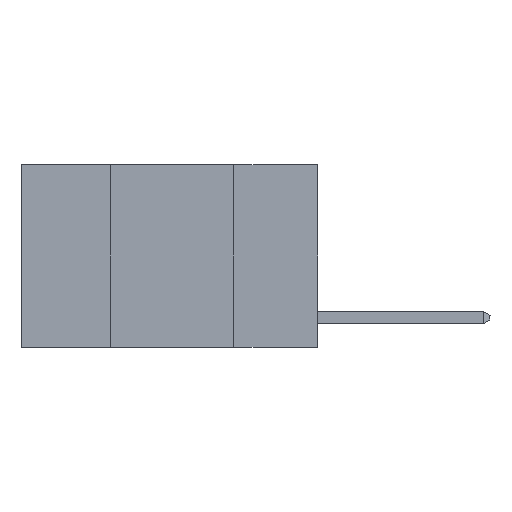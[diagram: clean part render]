
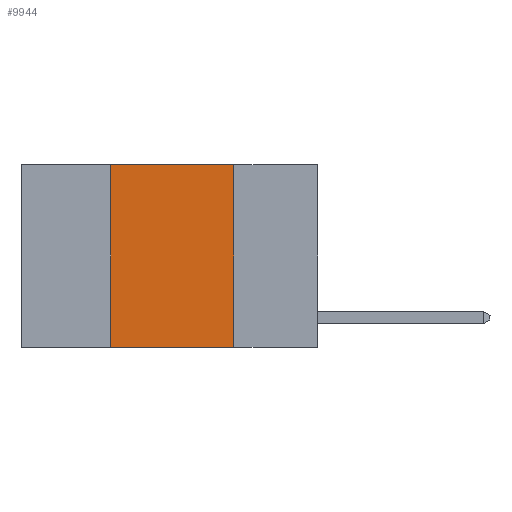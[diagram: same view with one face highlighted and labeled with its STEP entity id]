
A CAD part, left-side view. The second image highlights one B-rep face of the part: STEP entity #9944.
In plain terms, the highlighted planar face has unit normal (-1, 0, 0).
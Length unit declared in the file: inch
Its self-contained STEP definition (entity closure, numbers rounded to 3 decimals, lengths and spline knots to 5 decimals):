
#78 = EDGE_CURVE ( 'NONE', #9861, #7901, #6648, .T. ) ;
#279 = ORIENTED_EDGE ( 'NONE', *, *, #1181, .T. ) ;
#716 = CARTESIAN_POINT ( 'NONE',  ( 0., 0.6, 0. ) ) ;
#1181 = EDGE_CURVE ( 'NONE', #4732, #7901, #4963, .T. ) ;
#1214 = PLANE ( 'NONE',  #4737 ) ;
#1328 = EDGE_LOOP ( 'NONE', ( #4521, #8179, #10291, #279 ) ) ;
#1465 = CARTESIAN_POINT ( 'NONE',  ( 0., 0.42, -0.37 ) ) ;
#1724 = DIRECTION ( 'NONE',  ( 0., -1., 0. ) ) ;
#1966 = DIRECTION ( 'NONE',  ( 0., 0., -1. ) ) ;
#2116 = DIRECTION ( 'NONE',  ( 1., 0., 0. ) ) ;
#2265 = EDGE_CURVE ( 'NONE', #4308, #9861, #6457, .T. ) ;
#2433 = VECTOR ( 'NONE', #10717, 39.37008 ) ;
#2721 = VECTOR ( 'NONE', #1724, 39.37008 ) ;
#3752 = VECTOR ( 'NONE', #5620, 39.37008 ) ;
#3989 = FACE_OUTER_BOUND ( 'NONE', #1328, .T. ) ;
#4106 = CARTESIAN_POINT ( 'NONE',  ( 0., 0.6, 0. ) ) ;
#4308 = VERTEX_POINT ( 'NONE', #8028 ) ;
#4517 = VECTOR ( 'NONE', #1966, 39.37008 ) ;
#4521 = ORIENTED_EDGE ( 'NONE', *, *, #78, .F. ) ;
#4732 = VERTEX_POINT ( 'NONE', #1465 ) ;
#4737 = AXIS2_PLACEMENT_3D ( 'NONE', #4106, #2116, #8637 ) ;
#4963 = LINE ( 'NONE', #9739, #2433 ) ;
#5620 = DIRECTION ( 'NONE',  ( 0., 0., 1. ) ) ;
#6457 = LINE ( 'NONE', #716, #2721 ) ;
#6528 = CARTESIAN_POINT ( 'NONE',  ( 0., 0.42, 0. ) ) ;
#6648 = LINE ( 'NONE', #10371, #4517 ) ;
#7449 = LINE ( 'NONE', #6528, #3752 ) ;
#7901 = VERTEX_POINT ( 'NONE', #11365 ) ;
#8028 = CARTESIAN_POINT ( 'NONE',  ( 0., 0.42, 0. ) ) ;
#8179 = ORIENTED_EDGE ( 'NONE', *, *, #2265, .F. ) ;
#8637 = DIRECTION ( 'NONE',  ( 0., 0., -1. ) ) ;
#9440 = EDGE_CURVE ( 'NONE', #4732, #4308, #7449, .T. ) ;
#9739 = CARTESIAN_POINT ( 'NONE',  ( 0., 0.6, -0.37 ) ) ;
#9861 = VERTEX_POINT ( 'NONE', #10215 ) ;
#9944 = ADVANCED_FACE ( 'NONE', ( #3989 ), #1214, .F. ) ;
#10215 = CARTESIAN_POINT ( 'NONE',  ( 0., 0.17, 0. ) ) ;
#10291 = ORIENTED_EDGE ( 'NONE', *, *, #9440, .F. ) ;
#10371 = CARTESIAN_POINT ( 'NONE',  ( 0., 0.17, 0. ) ) ;
#10717 = DIRECTION ( 'NONE',  ( 0., -1., 0. ) ) ;
#11365 = CARTESIAN_POINT ( 'NONE',  ( 0., 0.17, -0.37 ) ) ;
